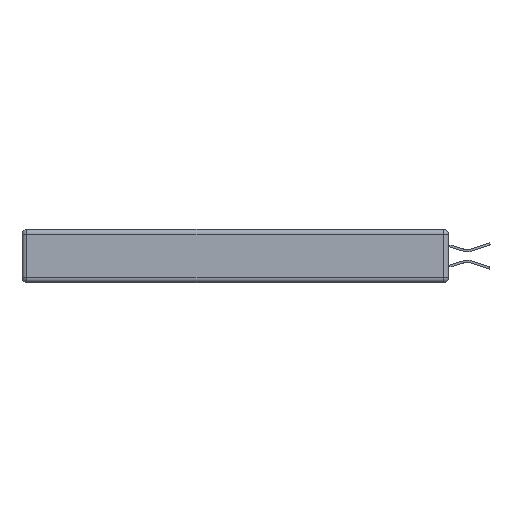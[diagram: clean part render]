
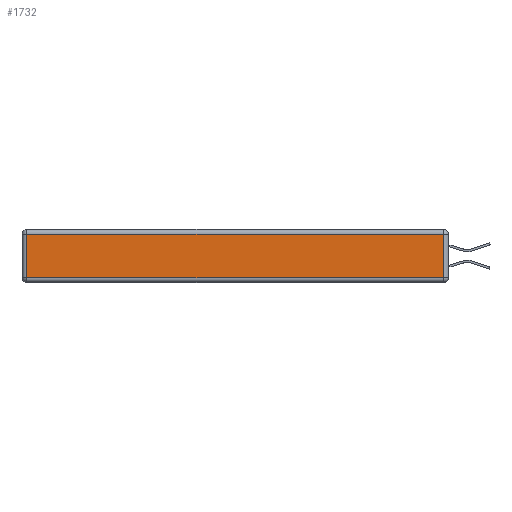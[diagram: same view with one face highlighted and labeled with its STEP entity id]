
A CAD part, left-side view. The second image highlights one B-rep face of the part: STEP entity #1732.
In plain terms, the highlighted planar face has unit normal (-1, 0, 0).
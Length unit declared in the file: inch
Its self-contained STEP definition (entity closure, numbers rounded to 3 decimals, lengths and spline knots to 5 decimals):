
#18 = DIRECTION ( 'NONE',  ( -1., 0., 0. ) ) ;
#275 = DIRECTION ( 'NONE',  ( 0., -1., 0. ) ) ;
#498 = DIRECTION ( 'NONE',  ( 0., 0., 1. ) ) ;
#557 = DIRECTION ( 'NONE',  ( 0., 1., 0. ) ) ;
#708 = ORIENTED_EDGE ( 'NONE', *, *, #7049, .T. ) ;
#948 = EDGE_CURVE ( 'NONE', #13026, #12720, #7450, .T. ) ;
#1732 = ADVANCED_FACE ( 'NONE', ( #8481 ), #12185, .T. ) ;
#2366 = VERTEX_POINT ( 'NONE', #10772 ) ;
#3290 = DIRECTION ( 'NONE',  ( 0., 0., 1. ) ) ;
#3674 = CARTESIAN_POINT ( 'NONE',  ( 0., 0., -0.313 ) ) ;
#4319 = ORIENTED_EDGE ( 'NONE', *, *, #948, .T. ) ;
#4538 = VECTOR ( 'NONE', #498, 39.37008 ) ;
#4956 = EDGE_LOOP ( 'NONE', ( #708, #4319, #13203, #9651 ) ) ;
#5126 = CARTESIAN_POINT ( 'NONE',  ( 0., 0.03, -0.313 ) ) ;
#5134 = LINE ( 'NONE', #7112, #11179 ) ;
#5893 = CARTESIAN_POINT ( 'NONE',  ( 0., 0.03, -0.343 ) ) ;
#6024 = VERTEX_POINT ( 'NONE', #7915 ) ;
#7049 = EDGE_CURVE ( 'NONE', #6024, #13026, #14213, .T. ) ;
#7112 = CARTESIAN_POINT ( 'NONE',  ( 0., 2.75, -0.03 ) ) ;
#7428 = VECTOR ( 'NONE', #7943, 39.37008 ) ;
#7450 = LINE ( 'NONE', #5893, #4538 ) ;
#7594 = EDGE_CURVE ( 'NONE', #12720, #2366, #5134, .T. ) ;
#7915 = CARTESIAN_POINT ( 'NONE',  ( 0., 2.72, -0.313 ) ) ;
#7943 = DIRECTION ( 'NONE',  ( 0., 0., -1. ) ) ;
#8481 = FACE_OUTER_BOUND ( 'NONE', #4956, .T. ) ;
#9651 = ORIENTED_EDGE ( 'NONE', *, *, #11656, .T. ) ;
#10357 = LINE ( 'NONE', #12318, #7428 ) ;
#10772 = CARTESIAN_POINT ( 'NONE',  ( 0., 2.72, -0.03 ) ) ;
#10928 = VECTOR ( 'NONE', #275, 39.37008 ) ;
#10939 = CARTESIAN_POINT ( 'NONE',  ( 0., 0., -0.343 ) ) ;
#11179 = VECTOR ( 'NONE', #557, 39.37008 ) ;
#11656 = EDGE_CURVE ( 'NONE', #2366, #6024, #10357, .T. ) ;
#12185 = PLANE ( 'NONE',  #12339 ) ;
#12318 = CARTESIAN_POINT ( 'NONE',  ( 0., 2.72, -0.343 ) ) ;
#12339 = AXIS2_PLACEMENT_3D ( 'NONE', #10939, #18, #3290 ) ;
#12720 = VERTEX_POINT ( 'NONE', #14251 ) ;
#13026 = VERTEX_POINT ( 'NONE', #5126 ) ;
#13203 = ORIENTED_EDGE ( 'NONE', *, *, #7594, .T. ) ;
#14213 = LINE ( 'NONE', #3674, #10928 ) ;
#14251 = CARTESIAN_POINT ( 'NONE',  ( 0., 0.03, -0.03 ) ) ;
